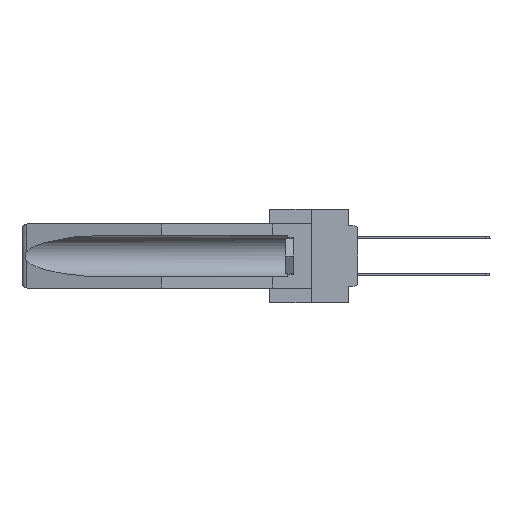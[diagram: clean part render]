
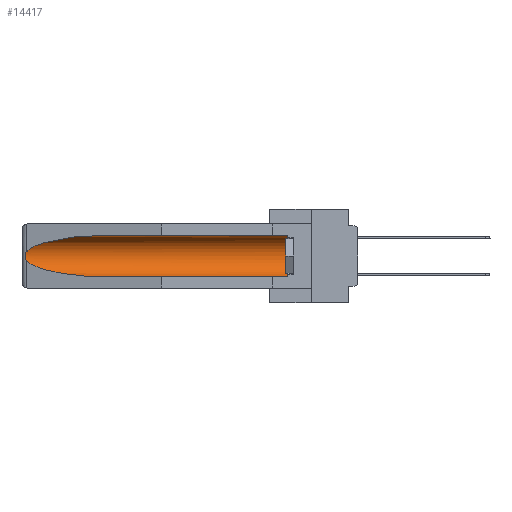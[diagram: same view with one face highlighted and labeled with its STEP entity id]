
A CAD part, left-side view. The second image highlights one B-rep face of the part: STEP entity #14417.
In plain terms, the highlighted cylindrical face has radius 2.857 mm (diameter 5.715 mm), a partial arc.
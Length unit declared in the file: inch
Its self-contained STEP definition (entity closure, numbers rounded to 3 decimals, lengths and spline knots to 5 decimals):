
#3 = CARTESIAN_POINT ( 'NONE',  ( 0.26537, 1.52718, -0.19328 ) ) ;
#394 = VERTEX_POINT ( 'NONE', #27304 ) ;
#451 = VECTOR ( 'NONE', #21098, 39.37008 ) ;
#548 = EDGE_CURVE ( 'NONE', #26517, #18035, #30235, .T. ) ;
#563 = ORIENTED_EDGE ( 'NONE', *, *, #27479, .T. ) ;
#1048 = CIRCLE ( 'NONE', #18371, 0.1125 ) ;
#1902 = DIRECTION ( 'NONE',  ( 0., 0., 1. ) ) ;
#2292 =( BOUNDED_CURVE ( )  B_SPLINE_CURVE ( 3, ( #22857, #23020, #4107, #27962 ),
 .UNSPECIFIED., .F., .F. ) 
 B_SPLINE_CURVE_WITH_KNOTS ( ( 4, 4 ),
 ( 0.1948, 1.5708 ),
 .UNSPECIFIED. ) 
 CURVE ( )  GEOMETRIC_REPRESENTATION_ITEM ( )  RATIONAL_B_SPLINE_CURVE ( ( 1., 0.848, 0.848, 1. ) ) 
 REPRESENTATION_ITEM ( '' )  );
#2361 = CARTESIAN_POINT ( 'NONE',  ( 0.155, -0.30754, -0.1715 ) ) ;
#3088 = ORIENTED_EDGE ( 'NONE', *, *, #6798, .T. ) ;
#4107 = CARTESIAN_POINT ( 'NONE',  ( 0.21114, 1.30732, -0.284 ) ) ;
#4168 = CARTESIAN_POINT ( 'NONE',  ( 0.155, 1.07973, -0.059 ) ) ;
#4278 = CARTESIAN_POINT ( 'NONE',  ( 0.155, 0.126, -0.059 ) ) ;
#4634 = ORIENTED_EDGE ( 'NONE', *, *, #5464, .T. ) ;
#4775 = CARTESIAN_POINT ( 'NONE',  ( 0.2675, 1.53308, -0.17534 ) ) ;
#5464 = EDGE_CURVE ( 'NONE', #19735, #29592, #2292, .T. ) ;
#6692 = DIRECTION ( 'NONE',  ( 0., 1., 0. ) ) ;
#6798 = EDGE_CURVE ( 'NONE', #394, #26517, #1048, .T. ) ;
#6948 = CARTESIAN_POINT ( 'NONE',  ( 0.26537, 1.52718, -0.14972 ) ) ;
#8487 = VERTEX_POINT ( 'NONE', #12750 ) ;
#8560 = DIRECTION ( 'NONE',  ( 0., 1., 0. ) ) ;
#9274 = CARTESIAN_POINT ( 'NONE',  ( 0.25451, 1.48313, -0.09465 ) ) ;
#10370 = CARTESIAN_POINT ( 'NONE',  ( 0.26537, 1.52718, -0.19328 ) ) ;
#11099 = EDGE_CURVE ( 'NONE', #394, #29592, #30251, .T. ) ;
#11302 = CARTESIAN_POINT ( 'NONE',  ( 0.26654, 1.53092, -0.15636 ) ) ;
#11908 = CARTESIAN_POINT ( 'NONE',  ( 0.2673, 1.5327, -0.16383 ) ) ;
#12750 = CARTESIAN_POINT ( 'NONE',  ( 0.26537, 1.52718, -0.14972 ) ) ;
#14086 = CARTESIAN_POINT ( 'NONE',  ( 0.26655, 1.53094, -0.18657 ) ) ;
#14137 =( BOUNDED_CURVE ( )  B_SPLINE_CURVE ( 3, ( #30191, #30498, #9274, #6948 ),
 .UNSPECIFIED., .F., .F. ) 
 B_SPLINE_CURVE_WITH_KNOTS ( ( 4, 4 ),
 ( 4.71239, 6.08839 ),
 .UNSPECIFIED. ) 
 CURVE ( )  GEOMETRIC_REPRESENTATION_ITEM ( )  RATIONAL_B_SPLINE_CURVE ( ( 1., 0.848, 0.848, 1. ) ) 
 REPRESENTATION_ITEM ( '' )  );
#14417 = ADVANCED_FACE ( 'NONE', ( #30400 ), #23123, .F. ) ;
#15384 = B_SPLINE_CURVE_WITH_KNOTS ( 'NONE', 3,
 ( #26025, #27878, #11302, #11908, #25723, #4775, #27723, #14086, #25403, #3 ),
 .UNSPECIFIED., .F., .F.,
 ( 4, 2, 2, 2, 4 ),
 ( 0., 0.00029, 0.00058, 0.00087, 0.00117 ),
 .UNSPECIFIED. ) ;
#16710 = ORIENTED_EDGE ( 'NONE', *, *, #11099, .F. ) ;
#17322 = EDGE_LOOP ( 'NONE', ( #563, #23362, #4634, #16710, #3088, #20036 ) ) ;
#18035 = VERTEX_POINT ( 'NONE', #4168 ) ;
#18371 = AXIS2_PLACEMENT_3D ( 'NONE', #24571, #20235, #26910 ) ;
#19735 = VERTEX_POINT ( 'NONE', #10370 ) ;
#19905 = VECTOR ( 'NONE', #8560, 39.37008 ) ;
#20036 = ORIENTED_EDGE ( 'NONE', *, *, #548, .T. ) ;
#20235 = DIRECTION ( 'NONE',  ( 0., -1., 0. ) ) ;
#20804 = CARTESIAN_POINT ( 'NONE',  ( 0.155, -0.30754, -0.284 ) ) ;
#21098 = DIRECTION ( 'NONE',  ( 0., 1., 0. ) ) ;
#21215 = EDGE_CURVE ( 'NONE', #8487, #19735, #15384, .T. ) ;
#22857 = CARTESIAN_POINT ( 'NONE',  ( 0.26537, 1.52718, -0.19328 ) ) ;
#23020 = CARTESIAN_POINT ( 'NONE',  ( 0.25451, 1.48313, -0.24835 ) ) ;
#23123 = CYLINDRICAL_SURFACE ( 'NONE', #23476, 0.1125 ) ;
#23362 = ORIENTED_EDGE ( 'NONE', *, *, #21215, .T. ) ;
#23476 = AXIS2_PLACEMENT_3D ( 'NONE', #2361, #6692, #1902 ) ;
#24571 = CARTESIAN_POINT ( 'NONE',  ( 0.155, 0.126, -0.1715 ) ) ;
#25403 = CARTESIAN_POINT ( 'NONE',  ( 0.26597, 1.5296, -0.19026 ) ) ;
#25479 = CARTESIAN_POINT ( 'NONE',  ( 0.155, 1.07973, -0.284 ) ) ;
#25723 = CARTESIAN_POINT ( 'NONE',  ( 0.2675, 1.53308, -0.16763 ) ) ;
#26025 = CARTESIAN_POINT ( 'NONE',  ( 0.26537, 1.52718, -0.14972 ) ) ;
#26517 = VERTEX_POINT ( 'NONE', #4278 ) ;
#26910 = DIRECTION ( 'NONE',  ( 0., 0., 1. ) ) ;
#27304 = CARTESIAN_POINT ( 'NONE',  ( 0.155, 0.126, -0.284 ) ) ;
#27479 = EDGE_CURVE ( 'NONE', #18035, #8487, #14137, .T. ) ;
#27723 = CARTESIAN_POINT ( 'NONE',  ( 0.2673, 1.53269, -0.17917 ) ) ;
#27878 = CARTESIAN_POINT ( 'NONE',  ( 0.26597, 1.52961, -0.15275 ) ) ;
#27962 = CARTESIAN_POINT ( 'NONE',  ( 0.155, 1.07973, -0.284 ) ) ;
#29592 = VERTEX_POINT ( 'NONE', #25479 ) ;
#30191 = CARTESIAN_POINT ( 'NONE',  ( 0.155, 1.07973, -0.059 ) ) ;
#30235 = LINE ( 'NONE', #30395, #451 ) ;
#30251 = LINE ( 'NONE', #20804, #19905 ) ;
#30395 = CARTESIAN_POINT ( 'NONE',  ( 0.155, -0.30754, -0.059 ) ) ;
#30400 = FACE_OUTER_BOUND ( 'NONE', #17322, .T. ) ;
#30498 = CARTESIAN_POINT ( 'NONE',  ( 0.21114, 1.30732, -0.059 ) ) ;
